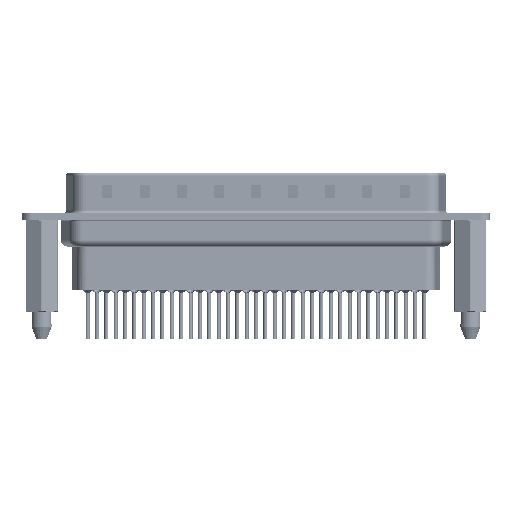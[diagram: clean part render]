
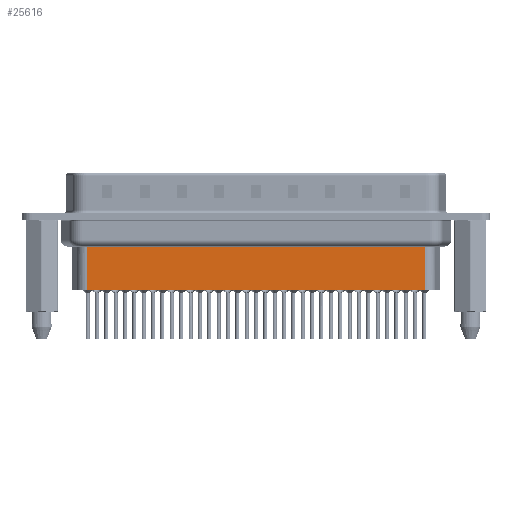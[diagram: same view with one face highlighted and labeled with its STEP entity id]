
A CAD part, front view. The second image highlights one B-rep face of the part: STEP entity #25616.
In plain terms, the highlighted planar face has unit normal (0, -1, 0).
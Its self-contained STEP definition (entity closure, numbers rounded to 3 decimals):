
#27 = ORIENTED_EDGE ( 'NONE', *, *, #15034, .F. ) ;
#630 = VECTOR ( 'NONE', #4425, 1000. ) ;
#1052 = VERTEX_POINT ( 'NONE', #3470 ) ;
#1727 = EDGE_CURVE ( 'NONE', #9383, #10461, #7151, .T. ) ;
#1733 = CARTESIAN_POINT ( 'NONE',  ( 6.706, -3.5, -10.95 ) ) ;
#1839 = DIRECTION ( 'NONE',  ( 1., 0., 0. ) ) ;
#1968 = EDGE_LOOP ( 'NONE', ( #27, #24430, #24832, #3271 ) ) ;
#3271 = ORIENTED_EDGE ( 'NONE', *, *, #1727, .F. ) ;
#3470 = CARTESIAN_POINT ( 'NONE',  ( 6.706, -3.5, -4.097 ) ) ;
#3660 = EDGE_CURVE ( 'NONE', #1052, #10461, #27893, .T. ) ;
#3765 = CARTESIAN_POINT ( 'NONE',  ( 56.794, -3.5, -10.95 ) ) ;
#4287 = DIRECTION ( 'NONE',  ( 0., -1., 0. ) ) ;
#4425 = DIRECTION ( 'NONE',  ( -1., 0., 0. ) ) ;
#4562 = CARTESIAN_POINT ( 'NONE',  ( 6.706, -3.5, -10.95 ) ) ;
#7151 = LINE ( 'NONE', #4562, #24651 ) ;
#8708 = AXIS2_PLACEMENT_3D ( 'NONE', #18457, #4287, #1839 ) ;
#9383 = VERTEX_POINT ( 'NONE', #3765 ) ;
#10198 = LINE ( 'NONE', #22262, #14551 ) ;
#10461 = VERTEX_POINT ( 'NONE', #1733 ) ;
#10897 = EDGE_CURVE ( 'NONE', #15176, #1052, #22174, .T. ) ;
#11755 = VECTOR ( 'NONE', #27572, 1000. ) ;
#14551 = VECTOR ( 'NONE', #14586, 1000. ) ;
#14586 = DIRECTION ( 'NONE',  ( 0., 0., -1. ) ) ;
#15034 = EDGE_CURVE ( 'NONE', #15176, #9383, #10198, .T. ) ;
#15176 = VERTEX_POINT ( 'NONE', #21058 ) ;
#16748 = DIRECTION ( 'NONE',  ( -1., 0., 0. ) ) ;
#18457 = CARTESIAN_POINT ( 'NONE',  ( 6.706, -3.5, -3.1 ) ) ;
#21058 = CARTESIAN_POINT ( 'NONE',  ( 56.794, -3.5, -4.097 ) ) ;
#22174 = LINE ( 'NONE', #31924, #630 ) ;
#22262 = CARTESIAN_POINT ( 'NONE',  ( 56.794, -3.5, -3.1 ) ) ;
#22550 = CARTESIAN_POINT ( 'NONE',  ( 6.706, -3.5, -3.1 ) ) ;
#24132 = PLANE ( 'NONE',  #8708 ) ;
#24430 = ORIENTED_EDGE ( 'NONE', *, *, #10897, .T. ) ;
#24651 = VECTOR ( 'NONE', #16748, 1000. ) ;
#24832 = ORIENTED_EDGE ( 'NONE', *, *, #3660, .T. ) ;
#25616 = ADVANCED_FACE ( 'NONE', ( #26093 ), #24132, .T. ) ;
#26093 = FACE_OUTER_BOUND ( 'NONE', #1968, .T. ) ;
#27572 = DIRECTION ( 'NONE',  ( 0., 0., -1. ) ) ;
#27893 = LINE ( 'NONE', #22550, #11755 ) ;
#31924 = CARTESIAN_POINT ( 'NONE',  ( 6.459, -3.5, -4.097 ) ) ;
